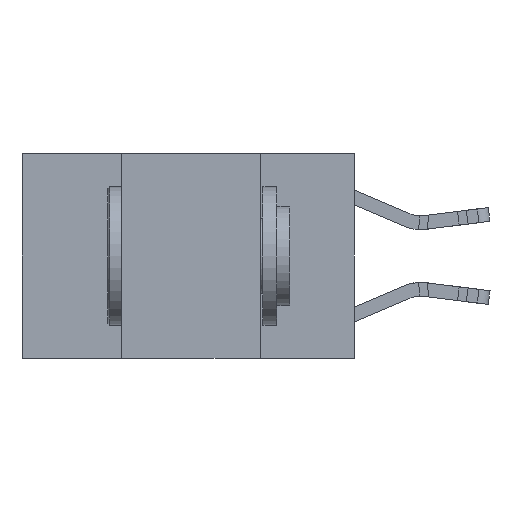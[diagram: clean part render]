
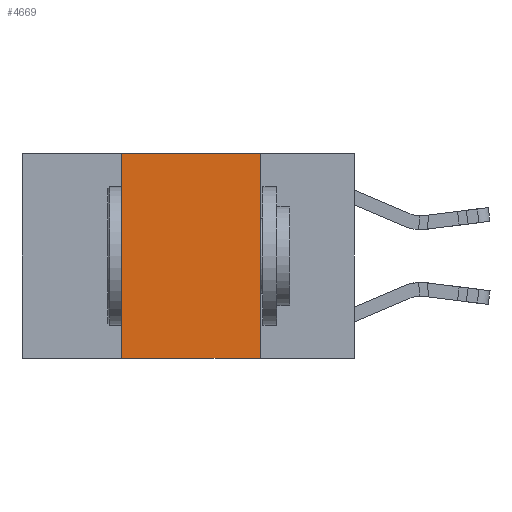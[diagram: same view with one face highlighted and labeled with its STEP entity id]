
A CAD part, left-side view. The second image highlights one B-rep face of the part: STEP entity #4669.
In plain terms, the highlighted planar face has unit normal (-1, 0, 0).
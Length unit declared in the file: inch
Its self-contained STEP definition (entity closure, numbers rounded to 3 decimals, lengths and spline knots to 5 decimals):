
#1129 = VECTOR ( 'NONE', #29837, 39.37008 ) ;
#1606 = ORIENTED_EDGE ( 'NONE', *, *, #22226, .F. ) ;
#2343 = LINE ( 'NONE', #19222, #14709 ) ;
#2638 = CARTESIAN_POINT ( 'NONE',  ( 0., 0.17, 0. ) ) ;
#3008 = VECTOR ( 'NONE', #27337, 39.37008 ) ;
#3595 = EDGE_CURVE ( 'NONE', #16317, #13816, #26623, .T. ) ;
#4551 = ORIENTED_EDGE ( 'NONE', *, *, #3595, .T. ) ;
#4669 = ADVANCED_FACE ( 'NONE', ( #21799 ), #17735, .F. ) ;
#5369 = DIRECTION ( 'NONE',  ( 0., 0., 1. ) ) ;
#6189 = DIRECTION ( 'NONE',  ( 0., 0., -1. ) ) ;
#6955 = ORIENTED_EDGE ( 'NONE', *, *, #24875, .F. ) ;
#7742 = CARTESIAN_POINT ( 'NONE',  ( 0., 0.42, 0. ) ) ;
#8809 = VERTEX_POINT ( 'NONE', #7742 ) ;
#10372 = ORIENTED_EDGE ( 'NONE', *, *, #20163, .F. ) ;
#13816 = VERTEX_POINT ( 'NONE', #21903 ) ;
#14070 = CARTESIAN_POINT ( 'NONE',  ( 0., 0.6, 0. ) ) ;
#14709 = VECTOR ( 'NONE', #5369, 39.37008 ) ;
#15413 = CARTESIAN_POINT ( 'NONE',  ( 0., 0.6, 0. ) ) ;
#16317 = VERTEX_POINT ( 'NONE', #19420 ) ;
#16402 = DIRECTION ( 'NONE',  ( 0., -1., 0. ) ) ;
#17735 = PLANE ( 'NONE',  #22212 ) ;
#18072 = LINE ( 'NONE', #14070, #29680 ) ;
#19222 = CARTESIAN_POINT ( 'NONE',  ( 0., 0.42, 0. ) ) ;
#19420 = CARTESIAN_POINT ( 'NONE',  ( 0., 0.42, -0.37 ) ) ;
#20075 = DIRECTION ( 'NONE',  ( 1., 0., 0. ) ) ;
#20163 = EDGE_CURVE ( 'NONE', #16317, #8809, #2343, .T. ) ;
#21543 = LINE ( 'NONE', #25031, #3008 ) ;
#21799 = FACE_OUTER_BOUND ( 'NONE', #26051, .T. ) ;
#21903 = CARTESIAN_POINT ( 'NONE',  ( 0., 0.17, -0.37 ) ) ;
#22212 = AXIS2_PLACEMENT_3D ( 'NONE', #15413, #20075, #6189 ) ;
#22226 = EDGE_CURVE ( 'NONE', #22473, #13816, #21543, .T. ) ;
#22473 = VERTEX_POINT ( 'NONE', #2638 ) ;
#24875 = EDGE_CURVE ( 'NONE', #8809, #22473, #18072, .T. ) ;
#25031 = CARTESIAN_POINT ( 'NONE',  ( 0., 0.17, 0. ) ) ;
#25263 = CARTESIAN_POINT ( 'NONE',  ( 0., 0.6, -0.37 ) ) ;
#26051 = EDGE_LOOP ( 'NONE', ( #1606, #6955, #10372, #4551 ) ) ;
#26623 = LINE ( 'NONE', #25263, #1129 ) ;
#27337 = DIRECTION ( 'NONE',  ( 0., 0., -1. ) ) ;
#29680 = VECTOR ( 'NONE', #16402, 39.37008 ) ;
#29837 = DIRECTION ( 'NONE',  ( 0., -1., 0. ) ) ;
